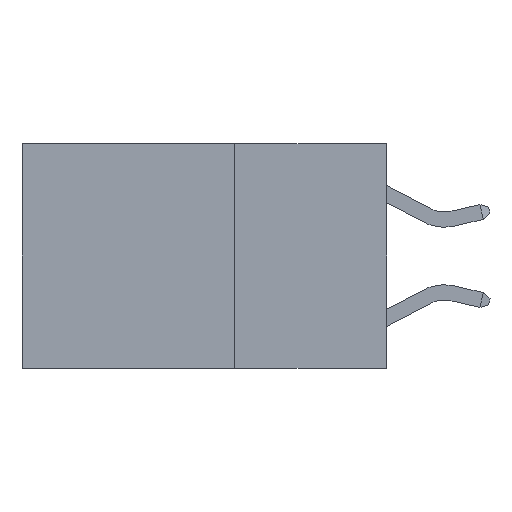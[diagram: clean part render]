
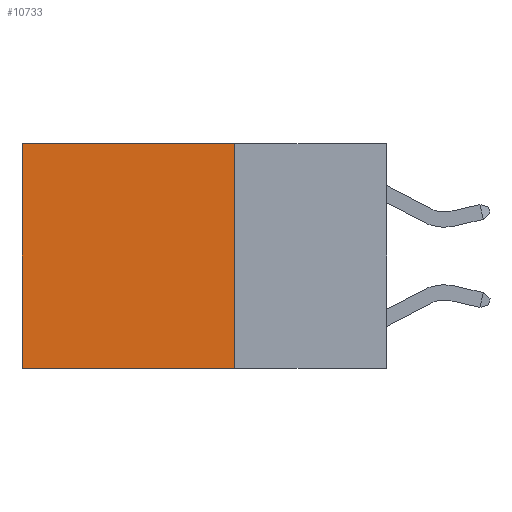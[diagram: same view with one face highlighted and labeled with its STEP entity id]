
A CAD part, left-side view. The second image highlights one B-rep face of the part: STEP entity #10733.
In plain terms, the highlighted planar face has unit normal (-1, 0, 0).
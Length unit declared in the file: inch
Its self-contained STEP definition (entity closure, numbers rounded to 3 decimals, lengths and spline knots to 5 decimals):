
#45 = ORIENTED_EDGE ( 'NONE', *, *, #3776, .T. ) ;
#132 = ORIENTED_EDGE ( 'NONE', *, *, #10608, .F. ) ;
#198 = ORIENTED_EDGE ( 'NONE', *, *, #3753, .F. ) ;
#210 = ORIENTED_EDGE ( 'NONE', *, *, #7241, .T. ) ;
#1204 = CARTESIAN_POINT ( 'NONE',  ( 0.2625, 0.25, 0. ) ) ;
#1593 = VECTOR ( 'NONE', #9947, 39.37008 ) ;
#1936 = EDGE_LOOP ( 'NONE', ( #45, #132, #198, #210 ) ) ;
#2138 = CARTESIAN_POINT ( 'NONE',  ( 0.2625, 0.6, -0.37 ) ) ;
#2146 = DIRECTION ( 'NONE',  ( 0., 0., -1. ) ) ;
#2573 = VERTEX_POINT ( 'NONE', #2138 ) ;
#2971 = CARTESIAN_POINT ( 'NONE',  ( 0.2625, 0.6, 0. ) ) ;
#3753 = EDGE_CURVE ( 'NONE', #8090, #10705, #6256, .T. ) ;
#3754 = DIRECTION ( 'NONE',  ( 0., 1., 0. ) ) ;
#3776 = EDGE_CURVE ( 'NONE', #8489, #2573, #6004, .T. ) ;
#4102 = LINE ( 'NONE', #7156, #4373 ) ;
#4373 = VECTOR ( 'NONE', #3754, 39.37008 ) ;
#4795 = CARTESIAN_POINT ( 'NONE',  ( 0.2625, 0.25, -0.37 ) ) ;
#4930 = CARTESIAN_POINT ( 'NONE',  ( 0.2625, 0.25, 0. ) ) ;
#5038 = FACE_OUTER_BOUND ( 'NONE', #1936, .T. ) ;
#5636 = PLANE ( 'NONE',  #8251 ) ;
#5811 = CARTESIAN_POINT ( 'NONE',  ( 0.2625, 0.6, 0. ) ) ;
#6004 = LINE ( 'NONE', #5811, #10169 ) ;
#6256 = LINE ( 'NONE', #4930, #1593 ) ;
#6597 = DIRECTION ( 'NONE',  ( 0., 0., -1. ) ) ;
#7156 = CARTESIAN_POINT ( 'NONE',  ( 0.2625, 0.25, -0.37 ) ) ;
#7241 = EDGE_CURVE ( 'NONE', #8090, #8489, #11212, .T. ) ;
#7281 = CARTESIAN_POINT ( 'NONE',  ( 0.2625, 0.25, 0. ) ) ;
#7346 = DIRECTION ( 'NONE',  ( 1., 0., 0. ) ) ;
#8090 = VERTEX_POINT ( 'NONE', #9299 ) ;
#8176 = DIRECTION ( 'NONE',  ( 0., 1., 0. ) ) ;
#8251 = AXIS2_PLACEMENT_3D ( 'NONE', #1204, #7346, #2146 ) ;
#8489 = VERTEX_POINT ( 'NONE', #2971 ) ;
#9061 = VECTOR ( 'NONE', #8176, 39.37008 ) ;
#9299 = CARTESIAN_POINT ( 'NONE',  ( 0.2625, 0.25, 0. ) ) ;
#9947 = DIRECTION ( 'NONE',  ( 0., 0., -1. ) ) ;
#10169 = VECTOR ( 'NONE', #6597, 39.37008 ) ;
#10608 = EDGE_CURVE ( 'NONE', #10705, #2573, #4102, .T. ) ;
#10705 = VERTEX_POINT ( 'NONE', #4795 ) ;
#10733 = ADVANCED_FACE ( 'NONE', ( #5038 ), #5636, .F. ) ;
#11212 = LINE ( 'NONE', #7281, #9061 ) ;
